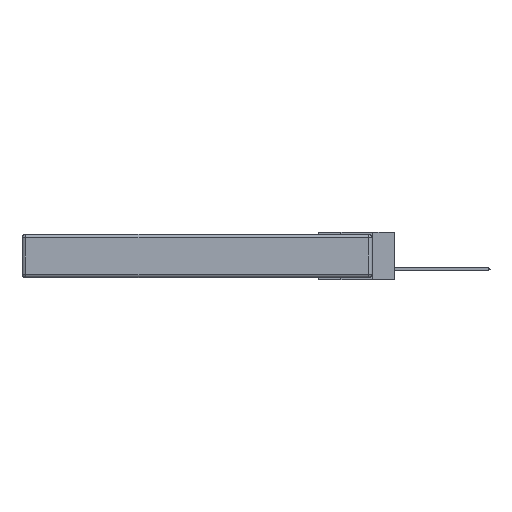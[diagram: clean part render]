
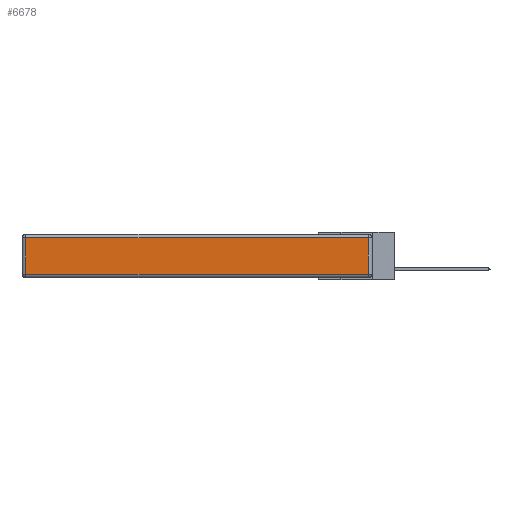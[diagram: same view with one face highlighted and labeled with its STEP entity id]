
A CAD part, left-side view. The second image highlights one B-rep face of the part: STEP entity #6678.
In plain terms, the highlighted planar face has unit normal (-1, 0, 0).
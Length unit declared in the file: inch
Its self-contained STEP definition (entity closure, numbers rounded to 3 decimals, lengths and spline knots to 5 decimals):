
#360 = EDGE_LOOP ( 'NONE', ( #29522, #25805, #13492, #25429 ) ) ;
#569 = VERTEX_POINT ( 'NONE', #19866 ) ;
#1300 = PLANE ( 'NONE',  #13661 ) ;
#1385 = EDGE_CURVE ( 'NONE', #8920, #4588, #4148, .T. ) ;
#1748 = CARTESIAN_POINT ( 'NONE',  ( 0., 0.03, -0.343 ) ) ;
#1849 = DIRECTION ( 'NONE',  ( 0., 0., 1. ) ) ;
#4148 = LINE ( 'NONE', #1748, #21215 ) ;
#4588 = VERTEX_POINT ( 'NONE', #32826 ) ;
#6678 = ADVANCED_FACE ( 'NONE', ( #32748 ), #1300, .T. ) ;
#7018 = LINE ( 'NONE', #13415, #8282 ) ;
#8282 = VECTOR ( 'NONE', #27153, 39.37008 ) ;
#8920 = VERTEX_POINT ( 'NONE', #16805 ) ;
#9990 = EDGE_CURVE ( 'NONE', #4588, #10275, #25425, .T. ) ;
#10120 = CARTESIAN_POINT ( 'NONE',  ( 0., 2.75, -0.03 ) ) ;
#10275 = VERTEX_POINT ( 'NONE', #11978 ) ;
#10356 = DIRECTION ( 'NONE',  ( 0., 1., 0. ) ) ;
#11784 = DIRECTION ( 'NONE',  ( 0., 0., 1. ) ) ;
#11978 = CARTESIAN_POINT ( 'NONE',  ( 0., 2.72, -0.03 ) ) ;
#12522 = VECTOR ( 'NONE', #10356, 39.37008 ) ;
#13415 = CARTESIAN_POINT ( 'NONE',  ( 0., 2.72, -0.343 ) ) ;
#13492 = ORIENTED_EDGE ( 'NONE', *, *, #9990, .T. ) ;
#13661 = AXIS2_PLACEMENT_3D ( 'NONE', #33242, #17128, #11784 ) ;
#16805 = CARTESIAN_POINT ( 'NONE',  ( 0., 0.03, -0.313 ) ) ;
#17128 = DIRECTION ( 'NONE',  ( -1., 0., 0. ) ) ;
#18980 = LINE ( 'NONE', #21626, #22717 ) ;
#19866 = CARTESIAN_POINT ( 'NONE',  ( 0., 2.72, -0.313 ) ) ;
#21215 = VECTOR ( 'NONE', #1849, 39.37008 ) ;
#21626 = CARTESIAN_POINT ( 'NONE',  ( 0., 0., -0.313 ) ) ;
#22717 = VECTOR ( 'NONE', #32297, 39.37008 ) ;
#25425 = LINE ( 'NONE', #10120, #12522 ) ;
#25429 = ORIENTED_EDGE ( 'NONE', *, *, #29923, .T. ) ;
#25805 = ORIENTED_EDGE ( 'NONE', *, *, #1385, .T. ) ;
#27153 = DIRECTION ( 'NONE',  ( 0., 0., -1. ) ) ;
#29522 = ORIENTED_EDGE ( 'NONE', *, *, #32020, .T. ) ;
#29923 = EDGE_CURVE ( 'NONE', #10275, #569, #7018, .T. ) ;
#32020 = EDGE_CURVE ( 'NONE', #569, #8920, #18980, .T. ) ;
#32297 = DIRECTION ( 'NONE',  ( 0., -1., 0. ) ) ;
#32748 = FACE_OUTER_BOUND ( 'NONE', #360, .T. ) ;
#32826 = CARTESIAN_POINT ( 'NONE',  ( 0., 0.03, -0.03 ) ) ;
#33242 = CARTESIAN_POINT ( 'NONE',  ( 0., 0., -0.343 ) ) ;
